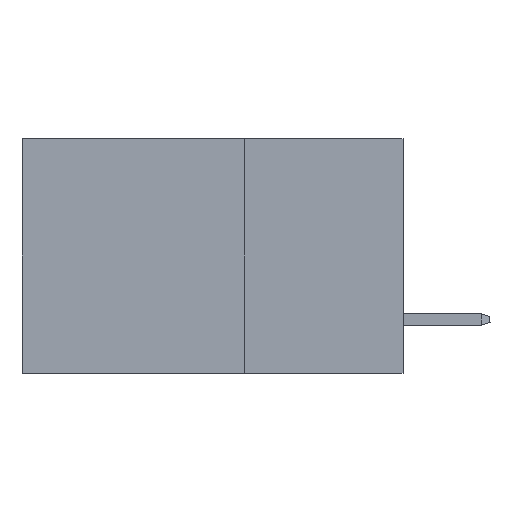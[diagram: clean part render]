
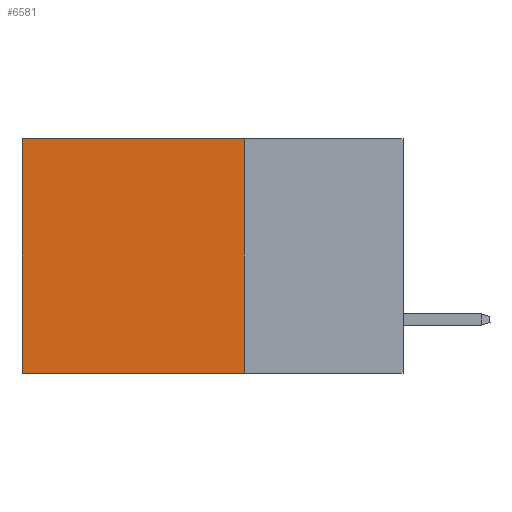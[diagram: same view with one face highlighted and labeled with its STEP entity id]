
A CAD part, left-side view. The second image highlights one B-rep face of the part: STEP entity #6581.
In plain terms, the highlighted planar face has unit normal (-1, 0, 0).
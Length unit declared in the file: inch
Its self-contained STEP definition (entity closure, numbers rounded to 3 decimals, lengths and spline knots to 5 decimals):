
#332 = PLANE ( 'NONE',  #4241 ) ;
#926 = DIRECTION ( 'NONE',  ( 1., 0., 0. ) ) ;
#1023 = EDGE_CURVE ( 'NONE', #8317, #10930, #16898, .T. ) ;
#3677 = CARTESIAN_POINT ( 'NONE',  ( 0.2875, 0.6, -0.37 ) ) ;
#4241 = AXIS2_PLACEMENT_3D ( 'NONE', #22067, #926, #23968 ) ;
#4278 = VERTEX_POINT ( 'NONE', #3677 ) ;
#6137 = FACE_OUTER_BOUND ( 'NONE', #10233, .T. ) ;
#6581 = ADVANCED_FACE ( 'NONE', ( #6137 ), #332, .F. ) ;
#7536 = CARTESIAN_POINT ( 'NONE',  ( 0.2875, 0.25, 0. ) ) ;
#8317 = VERTEX_POINT ( 'NONE', #23636 ) ;
#8457 = CARTESIAN_POINT ( 'NONE',  ( 0.2875, 0.6, 0. ) ) ;
#8813 = CARTESIAN_POINT ( 'NONE',  ( 0.2875, 0.25, -0.37 ) ) ;
#10233 = EDGE_LOOP ( 'NONE', ( #12910, #10668, #16049, #17115 ) ) ;
#10668 = ORIENTED_EDGE ( 'NONE', *, *, #12573, .F. ) ;
#10930 = VERTEX_POINT ( 'NONE', #8457 ) ;
#11328 = DIRECTION ( 'NONE',  ( 0., 0., -1. ) ) ;
#12210 = LINE ( 'NONE', #8813, #22893 ) ;
#12573 = EDGE_CURVE ( 'NONE', #19586, #4278, #12210, .T. ) ;
#12582 = CARTESIAN_POINT ( 'NONE',  ( 0.2875, 0.25, -0.37 ) ) ;
#12812 = VECTOR ( 'NONE', #11328, 39.37008 ) ;
#12910 = ORIENTED_EDGE ( 'NONE', *, *, #24571, .T. ) ;
#13227 = CARTESIAN_POINT ( 'NONE',  ( 0.2875, 0.6, 0. ) ) ;
#16049 = ORIENTED_EDGE ( 'NONE', *, *, #18520, .F. ) ;
#16898 = LINE ( 'NONE', #24566, #20107 ) ;
#17115 = ORIENTED_EDGE ( 'NONE', *, *, #1023, .T. ) ;
#17122 = LINE ( 'NONE', #13227, #12812 ) ;
#18000 = DIRECTION ( 'NONE',  ( 0., 1., 0. ) ) ;
#18520 = EDGE_CURVE ( 'NONE', #8317, #19586, #18736, .T. ) ;
#18619 = DIRECTION ( 'NONE',  ( 0., 0., -1. ) ) ;
#18736 = LINE ( 'NONE', #7536, #21004 ) ;
#19586 = VERTEX_POINT ( 'NONE', #12582 ) ;
#20107 = VECTOR ( 'NONE', #20525, 39.37008 ) ;
#20525 = DIRECTION ( 'NONE',  ( 0., 1., 0. ) ) ;
#21004 = VECTOR ( 'NONE', #18619, 39.37008 ) ;
#22067 = CARTESIAN_POINT ( 'NONE',  ( 0.2875, 0.25, 0. ) ) ;
#22893 = VECTOR ( 'NONE', #18000, 39.37008 ) ;
#23636 = CARTESIAN_POINT ( 'NONE',  ( 0.2875, 0.25, 0. ) ) ;
#23968 = DIRECTION ( 'NONE',  ( 0., 0., -1. ) ) ;
#24566 = CARTESIAN_POINT ( 'NONE',  ( 0.2875, 0.25, 0. ) ) ;
#24571 = EDGE_CURVE ( 'NONE', #10930, #4278, #17122, .T. ) ;
